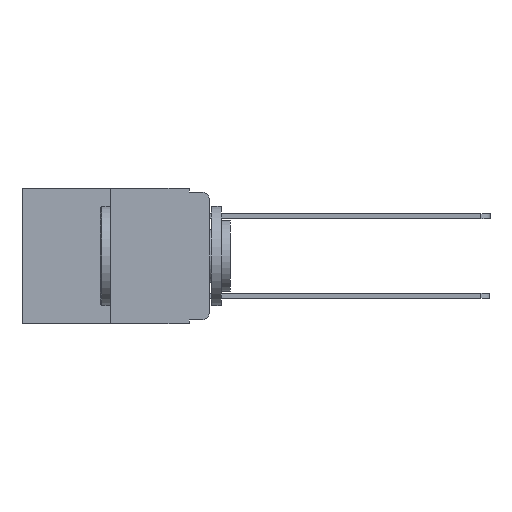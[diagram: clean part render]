
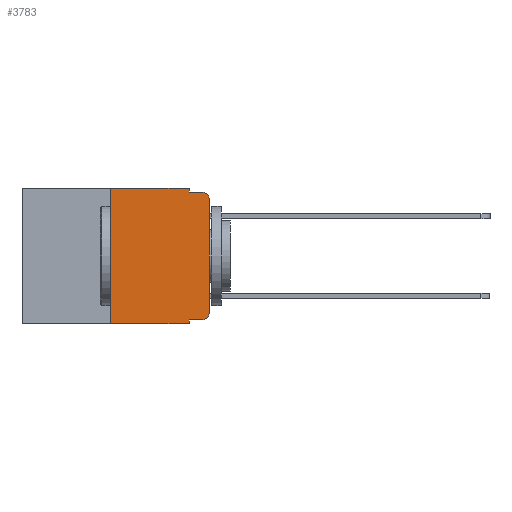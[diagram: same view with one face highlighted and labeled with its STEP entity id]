
A CAD part, left-side view. The second image highlights one B-rep face of the part: STEP entity #3783.
In plain terms, the highlighted planar face has unit normal (-1, 0, 0).
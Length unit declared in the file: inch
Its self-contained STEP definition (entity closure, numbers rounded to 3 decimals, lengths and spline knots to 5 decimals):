
#191 = EDGE_CURVE ( 'NONE', #15614, #990, #2260, .T. ) ;
#990 = VERTEX_POINT ( 'NONE', #16090 ) ;
#1191 = VERTEX_POINT ( 'NONE', #13847 ) ;
#1214 = EDGE_CURVE ( 'NONE', #11136, #1191, #12937, .T. ) ;
#1545 = DIRECTION ( 'NONE',  ( 0., 0., -1. ) ) ;
#1582 = VERTEX_POINT ( 'NONE', #13167 ) ;
#2075 = CARTESIAN_POINT ( 'NONE',  ( 0., 0.25, 0. ) ) ;
#2260 = LINE ( 'NONE', #7756, #15273 ) ;
#2533 = EDGE_CURVE ( 'NONE', #11136, #990, #9774, .T. ) ;
#3143 = VERTEX_POINT ( 'NONE', #2075 ) ;
#3592 = LINE ( 'NONE', #8586, #20554 ) ;
#3725 = CARTESIAN_POINT ( 'NONE',  ( 0., 0., 0. ) ) ;
#3783 = ADVANCED_FACE ( 'NONE', ( #9400 ), #13582, .F. ) ;
#3806 = CARTESIAN_POINT ( 'NONE',  ( 0., 0.25, -0.343 ) ) ;
#3861 = VERTEX_POINT ( 'NONE', #3909 ) ;
#3909 = CARTESIAN_POINT ( 'NONE',  ( 0., 0.02, -0.01 ) ) ;
#4010 = ORIENTED_EDGE ( 'NONE', *, *, #7289, .F. ) ;
#4373 = DIRECTION ( 'NONE',  ( 0., -1., 0. ) ) ;
#4459 = CARTESIAN_POINT ( 'NONE',  ( 0., 0.051, -0.01 ) ) ;
#4574 = ORIENTED_EDGE ( 'NONE', *, *, #6761, .F. ) ;
#4781 = DIRECTION ( 'NONE',  ( -1., 0., 0. ) ) ;
#5041 = EDGE_CURVE ( 'NONE', #15614, #3143, #15207, .T. ) ;
#5081 = VERTEX_POINT ( 'NONE', #20068 ) ;
#5185 = CARTESIAN_POINT ( 'NONE',  ( 0., 0.051, -0.01 ) ) ;
#5301 = VECTOR ( 'NONE', #18066, 39.37008 ) ;
#5306 = DIRECTION ( 'NONE',  ( 0., 0., -1. ) ) ;
#5329 = VECTOR ( 'NONE', #9761, 39.37008 ) ;
#5477 = VERTEX_POINT ( 'NONE', #17775 ) ;
#5644 = ORIENTED_EDGE ( 'NONE', *, *, #191, .T. ) ;
#6335 = VECTOR ( 'NONE', #16019, 39.37008 ) ;
#6453 = VECTOR ( 'NONE', #20010, 39.37008 ) ;
#6761 = EDGE_CURVE ( 'NONE', #3143, #1582, #18363, .T. ) ;
#7047 = CARTESIAN_POINT ( 'NONE',  ( 0., 0.051, -0.333 ) ) ;
#7289 = EDGE_CURVE ( 'NONE', #1582, #16193, #3592, .T. ) ;
#7350 = AXIS2_PLACEMENT_3D ( 'NONE', #18357, #8577, #19954 ) ;
#7464 = ORIENTED_EDGE ( 'NONE', *, *, #9498, .T. ) ;
#7756 = CARTESIAN_POINT ( 'NONE',  ( 0., 0.473, -0.343 ) ) ;
#8051 = CARTESIAN_POINT ( 'NONE',  ( 0., 0.051, 0. ) ) ;
#8380 = EDGE_CURVE ( 'NONE', #16193, #3861, #18825, .T. ) ;
#8577 = DIRECTION ( 'NONE',  ( -1., 0., 0. ) ) ;
#8586 = CARTESIAN_POINT ( 'NONE',  ( 0., 0.051, 0. ) ) ;
#9009 = ORIENTED_EDGE ( 'NONE', *, *, #5041, .F. ) ;
#9194 = EDGE_LOOP ( 'NONE', ( #14677, #7464, #16203, #4010, #4574, #9009, #5644, #19182, #15455, #14190 ) ) ;
#9400 = FACE_OUTER_BOUND ( 'NONE', #9194, .T. ) ;
#9498 = EDGE_CURVE ( 'NONE', #5081, #3861, #10214, .T. ) ;
#9506 = DIRECTION ( 'NONE',  ( 0., -1., 0. ) ) ;
#9761 = DIRECTION ( 'NONE',  ( 0., 0., -1. ) ) ;
#9774 = LINE ( 'NONE', #8051, #5329 ) ;
#10007 = CARTESIAN_POINT ( 'NONE',  ( 0., 0.473, 0. ) ) ;
#10214 = CIRCLE ( 'NONE', #7350, 0.02 ) ;
#10354 = DIRECTION ( 'NONE',  ( 0., 0., 1. ) ) ;
#10374 = CARTESIAN_POINT ( 'NONE',  ( 0., 0.25, 0. ) ) ;
#11136 = VERTEX_POINT ( 'NONE', #7047 ) ;
#11591 = CIRCLE ( 'NONE', #12043, 0.02 ) ;
#12043 = AXIS2_PLACEMENT_3D ( 'NONE', #14698, #4781, #16342 ) ;
#12413 = VECTOR ( 'NONE', #4373, 39.37008 ) ;
#12815 = EDGE_CURVE ( 'NONE', #5477, #5081, #19042, .T. ) ;
#12937 = LINE ( 'NONE', #20549, #12413 ) ;
#13167 = CARTESIAN_POINT ( 'NONE',  ( 0., 0.051, 0. ) ) ;
#13582 = PLANE ( 'NONE',  #20685 ) ;
#13847 = CARTESIAN_POINT ( 'NONE',  ( 0., 0.02, -0.333 ) ) ;
#14190 = ORIENTED_EDGE ( 'NONE', *, *, #21810, .T. ) ;
#14677 = ORIENTED_EDGE ( 'NONE', *, *, #12815, .T. ) ;
#14698 = CARTESIAN_POINT ( 'NONE',  ( 0., 0.02, -0.313 ) ) ;
#15198 = DIRECTION ( 'NONE',  ( 1., 0., 0. ) ) ;
#15207 = LINE ( 'NONE', #10374, #6453 ) ;
#15273 = VECTOR ( 'NONE', #9506, 39.37008 ) ;
#15455 = ORIENTED_EDGE ( 'NONE', *, *, #1214, .T. ) ;
#15614 = VERTEX_POINT ( 'NONE', #3806 ) ;
#16019 = DIRECTION ( 'NONE',  ( 0., -1., 0. ) ) ;
#16090 = CARTESIAN_POINT ( 'NONE',  ( 0., 0.051, -0.343 ) ) ;
#16193 = VERTEX_POINT ( 'NONE', #5185 ) ;
#16203 = ORIENTED_EDGE ( 'NONE', *, *, #8380, .F. ) ;
#16342 = DIRECTION ( 'NONE',  ( 0., 0., -1. ) ) ;
#17775 = CARTESIAN_POINT ( 'NONE',  ( 0., 0., -0.313 ) ) ;
#18066 = DIRECTION ( 'NONE',  ( 0., -1., 0. ) ) ;
#18357 = CARTESIAN_POINT ( 'NONE',  ( 0., 0.02, -0.03 ) ) ;
#18363 = LINE ( 'NONE', #10007, #5301 ) ;
#18542 = VECTOR ( 'NONE', #10354, 39.37008 ) ;
#18825 = LINE ( 'NONE', #4459, #6335 ) ;
#19042 = LINE ( 'NONE', #3725, #18542 ) ;
#19182 = ORIENTED_EDGE ( 'NONE', *, *, #2533, .F. ) ;
#19954 = DIRECTION ( 'NONE',  ( 0., 0., -1. ) ) ;
#20010 = DIRECTION ( 'NONE',  ( 0., 0., 1. ) ) ;
#20068 = CARTESIAN_POINT ( 'NONE',  ( 0., 0., -0.03 ) ) ;
#20549 = CARTESIAN_POINT ( 'NONE',  ( 0., 0.051, -0.333 ) ) ;
#20554 = VECTOR ( 'NONE', #1545, 39.37008 ) ;
#20685 = AXIS2_PLACEMENT_3D ( 'NONE', #21520, #15198, #5306 ) ;
#21520 = CARTESIAN_POINT ( 'NONE',  ( 0., 0.473, 0. ) ) ;
#21810 = EDGE_CURVE ( 'NONE', #1191, #5477, #11591, .T. ) ;
